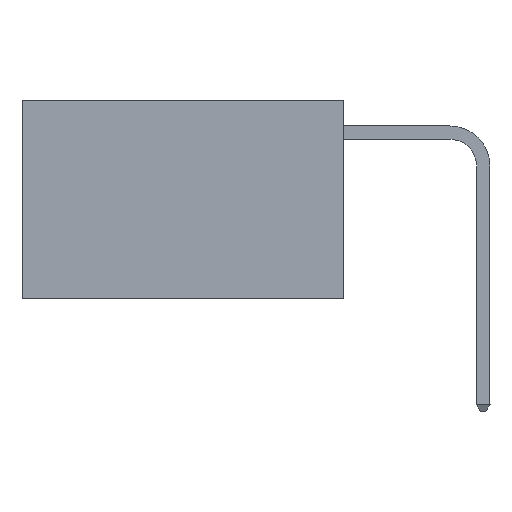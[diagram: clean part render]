
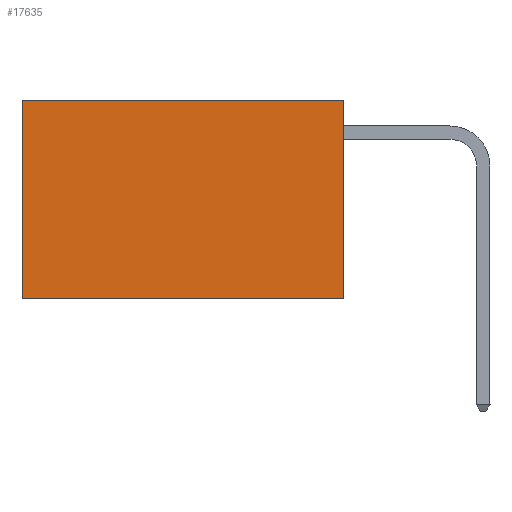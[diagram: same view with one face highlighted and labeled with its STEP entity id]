
A CAD part, left-side view. The second image highlights one B-rep face of the part: STEP entity #17635.
In plain terms, the highlighted planar face has unit normal (-1, 0, 0).
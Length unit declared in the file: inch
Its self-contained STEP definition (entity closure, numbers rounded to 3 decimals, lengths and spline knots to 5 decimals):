
#63 = PLANE ( 'NONE',  #5288 ) ;
#177 = EDGE_CURVE ( 'NONE', #2576, #4980, #23314, .T. ) ;
#480 = DIRECTION ( 'NONE',  ( 0., 0., -1. ) ) ;
#1076 = LINE ( 'NONE', #21418, #17356 ) ;
#1245 = EDGE_CURVE ( 'NONE', #4980, #23205, #1076, .T. ) ;
#1287 = LINE ( 'NONE', #9062, #12052 ) ;
#2198 = DIRECTION ( 'NONE',  ( 0., 0., -1. ) ) ;
#2576 = VERTEX_POINT ( 'NONE', #23474 ) ;
#3522 = ORIENTED_EDGE ( 'NONE', *, *, #1245, .F. ) ;
#4601 = ORIENTED_EDGE ( 'NONE', *, *, #17314, .T. ) ;
#4980 = VERTEX_POINT ( 'NONE', #10656 ) ;
#5288 = AXIS2_PLACEMENT_3D ( 'NONE', #23272, #14984, #2198 ) ;
#6978 = ORIENTED_EDGE ( 'NONE', *, *, #177, .F. ) ;
#8173 = VERTEX_POINT ( 'NONE', #15725 ) ;
#8914 = CARTESIAN_POINT ( 'NONE',  ( 0.2625, 0.6, -0.37 ) ) ;
#9062 = CARTESIAN_POINT ( 'NONE',  ( 0.2625, 0., 0. ) ) ;
#9802 = ORIENTED_EDGE ( 'NONE', *, *, #25341, .T. ) ;
#10656 = CARTESIAN_POINT ( 'NONE',  ( 0.2625, 0., -0.37 ) ) ;
#10857 = DIRECTION ( 'NONE',  ( 0., 1., 0. ) ) ;
#11227 = DIRECTION ( 'NONE',  ( 0., 1., 0. ) ) ;
#12052 = VECTOR ( 'NONE', #11227, 39.37008 ) ;
#12897 = VECTOR ( 'NONE', #480, 39.37008 ) ;
#12900 = VECTOR ( 'NONE', #24579, 39.37008 ) ;
#13317 = CARTESIAN_POINT ( 'NONE',  ( 0.2625, 0.6, 0. ) ) ;
#14984 = DIRECTION ( 'NONE',  ( 1., 0., 0. ) ) ;
#15725 = CARTESIAN_POINT ( 'NONE',  ( 0.2625, 0.6, 0. ) ) ;
#17314 = EDGE_CURVE ( 'NONE', #2576, #8173, #1287, .T. ) ;
#17356 = VECTOR ( 'NONE', #10857, 39.37008 ) ;
#17635 = ADVANCED_FACE ( 'NONE', ( #20829 ), #63, .F. ) ;
#19063 = LINE ( 'NONE', #13317, #12897 ) ;
#20829 = FACE_OUTER_BOUND ( 'NONE', #25646, .T. ) ;
#21418 = CARTESIAN_POINT ( 'NONE',  ( 0.2625, 0., -0.37 ) ) ;
#23205 = VERTEX_POINT ( 'NONE', #8914 ) ;
#23272 = CARTESIAN_POINT ( 'NONE',  ( 0.2625, 0., 0. ) ) ;
#23314 = LINE ( 'NONE', #26712, #12900 ) ;
#23474 = CARTESIAN_POINT ( 'NONE',  ( 0.2625, 0., 0. ) ) ;
#24579 = DIRECTION ( 'NONE',  ( 0., 0., -1. ) ) ;
#25341 = EDGE_CURVE ( 'NONE', #8173, #23205, #19063, .T. ) ;
#25646 = EDGE_LOOP ( 'NONE', ( #9802, #3522, #6978, #4601 ) ) ;
#26712 = CARTESIAN_POINT ( 'NONE',  ( 0.2625, 0., 0. ) ) ;
